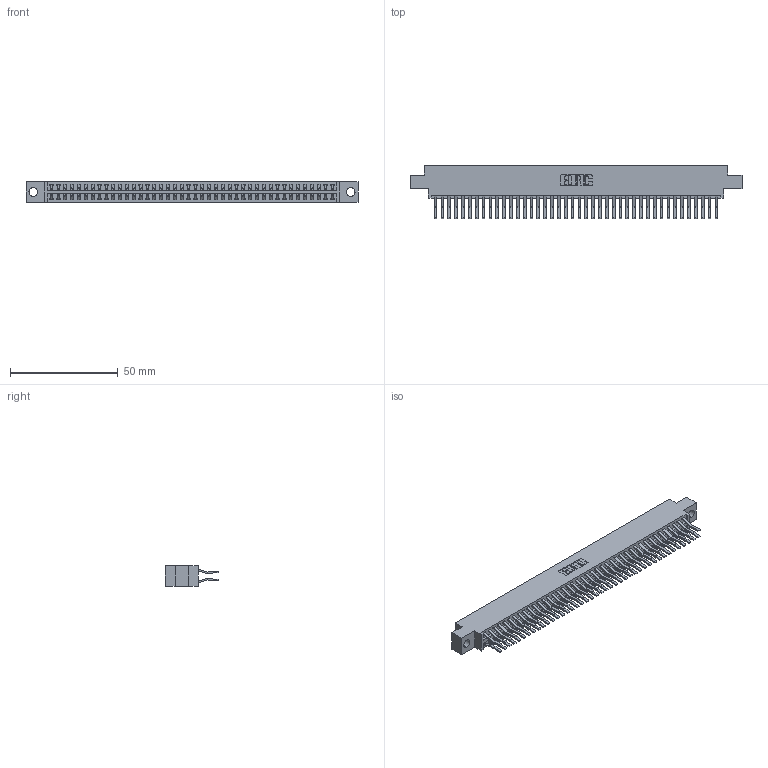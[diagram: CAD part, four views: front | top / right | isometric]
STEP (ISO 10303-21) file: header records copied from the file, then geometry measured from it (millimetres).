
FILE_DESCRIPTION (( 'STEP AP203' ), '1' );
FILE_NAME ('346-084-560-804.STEP', '2022-05-25T21:19:42', ( '' ), ( '' ), 'SwSTEP 2.0', 'SolidWorks 2020', '' );
FILE_SCHEMA (( 'CONFIG_CONTROL_DESIGN' ));
Length unit declared in the file: inch
Products named in the file (3): 346 Part_0.170 Offset - 0.156 Dia-TH; 345-292-001_560 Tail; 346-084-560-804
Assembly tree (85 placements, depth 2):
  346-084-560-804
    346 Part_0.170 Offset - 0.156 Dia-TH
    345-292-001_560 Tail  x84
Bounding box: 153.92 x 24.78 x 9.4 mm (x, y, z)
Volume: 15299.5 mm3; surface area: 22526.7 mm2
Topology: 85 solids, 85 shells, 4676 faces, 13901 edges, 9154 vertices
Faces by surface type: plane 3034, cylinder 1642
Entity records: 28049 total; most frequent: CARTESIAN_POINT 4630, ORIENTED_EDGE 4562, DIRECTION 4133, EDGE_CURVE 2281, LINE 1977, VECTOR 1977, VERTEX_POINT 1518, AXIS2_PLACEMENT_3D 1078
